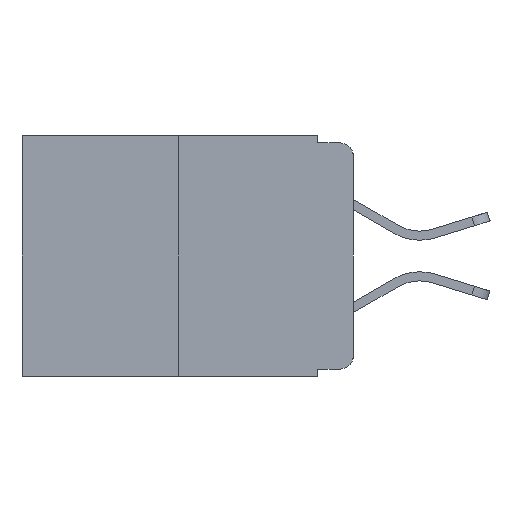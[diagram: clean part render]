
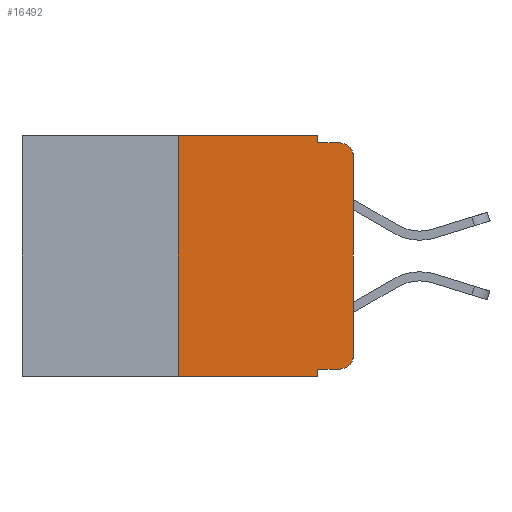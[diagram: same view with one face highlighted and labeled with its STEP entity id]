
A CAD part, left-side view. The second image highlights one B-rep face of the part: STEP entity #16492.
In plain terms, the highlighted planar face has unit normal (-1, 0, 0).
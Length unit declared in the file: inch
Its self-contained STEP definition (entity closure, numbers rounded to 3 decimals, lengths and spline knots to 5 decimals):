
#36 = VERTEX_POINT ( 'NONE', #6370 ) ;
#94 = DIRECTION ( 'NONE',  ( 0., -1., 0. ) ) ;
#273 = LINE ( 'NONE', #22919, #15031 ) ;
#414 = DIRECTION ( 'NONE',  ( 0., 0., 1. ) ) ;
#1648 = EDGE_CURVE ( 'NONE', #11393, #10844, #273, .T. ) ;
#1889 = EDGE_CURVE ( 'NONE', #9114, #8781, #11661, .T. ) ;
#2621 = EDGE_CURVE ( 'NONE', #20983, #8692, #7535, .T. ) ;
#2683 = ORIENTED_EDGE ( 'NONE', *, *, #15283, .F. ) ;
#3445 = PLANE ( 'NONE',  #17469 ) ;
#3870 = CARTESIAN_POINT ( 'NONE',  ( 0., 0.02, -0.333 ) ) ;
#4636 = DIRECTION ( 'NONE',  ( 0., 0., -1. ) ) ;
#5311 = AXIS2_PLACEMENT_3D ( 'NONE', #5682, #7785, #19036 ) ;
#5682 = CARTESIAN_POINT ( 'NONE',  ( 0., 0.02, -0.313 ) ) ;
#5916 = ORIENTED_EDGE ( 'NONE', *, *, #8315, .F. ) ;
#6162 = LINE ( 'NONE', #13438, #12718 ) ;
#6370 = CARTESIAN_POINT ( 'NONE',  ( 0., 0.051, -0.333 ) ) ;
#6625 = EDGE_CURVE ( 'NONE', #36, #10844, #10300, .T. ) ;
#6640 = ORIENTED_EDGE ( 'NONE', *, *, #12602, .F. ) ;
#7273 = CARTESIAN_POINT ( 'NONE',  ( 0., 0.473, 0. ) ) ;
#7356 = CARTESIAN_POINT ( 'NONE',  ( 0., 0.051, -0.01 ) ) ;
#7535 = LINE ( 'NONE', #22982, #11727 ) ;
#7785 = DIRECTION ( 'NONE',  ( -1., 0., 0. ) ) ;
#7858 = CARTESIAN_POINT ( 'NONE',  ( 0., 0., 0. ) ) ;
#7946 = DIRECTION ( 'NONE',  ( 0., -1., 0. ) ) ;
#8080 = ORIENTED_EDGE ( 'NONE', *, *, #1648, .T. ) ;
#8315 = EDGE_CURVE ( 'NONE', #11393, #20983, #23577, .T. ) ;
#8424 = ORIENTED_EDGE ( 'NONE', *, *, #2621, .F. ) ;
#8571 = CARTESIAN_POINT ( 'NONE',  ( 0., 0.051, -0.01 ) ) ;
#8614 = VERTEX_POINT ( 'NONE', #7356 ) ;
#8692 = VERTEX_POINT ( 'NONE', #10287 ) ;
#8781 = VERTEX_POINT ( 'NONE', #16011 ) ;
#9114 = VERTEX_POINT ( 'NONE', #21158 ) ;
#10287 = CARTESIAN_POINT ( 'NONE',  ( 0., 0.051, 0. ) ) ;
#10300 = LINE ( 'NONE', #21579, #15223 ) ;
#10808 = EDGE_CURVE ( 'NONE', #15470, #18124, #13994, .T. ) ;
#10844 = VERTEX_POINT ( 'NONE', #22866 ) ;
#11393 = VERTEX_POINT ( 'NONE', #18338 ) ;
#11661 = CIRCLE ( 'NONE', #14442, 0.02 ) ;
#11727 = VECTOR ( 'NONE', #94, 39.37008 ) ;
#11922 = DIRECTION ( 'NONE',  ( 0., 0., 1. ) ) ;
#12444 = ORIENTED_EDGE ( 'NONE', *, *, #10808, .T. ) ;
#12506 = LINE ( 'NONE', #8571, #15147 ) ;
#12602 = EDGE_CURVE ( 'NONE', #8614, #8781, #12506, .T. ) ;
#12718 = VECTOR ( 'NONE', #17678, 39.37008 ) ;
#12773 = VECTOR ( 'NONE', #414, 39.37008 ) ;
#12774 = DIRECTION ( 'NONE',  ( 0., -1., 0. ) ) ;
#13438 = CARTESIAN_POINT ( 'NONE',  ( 0., 0.051, 0. ) ) ;
#13825 = ORIENTED_EDGE ( 'NONE', *, *, #6625, .F. ) ;
#13994 = CIRCLE ( 'NONE', #5311, 0.02 ) ;
#14346 = CARTESIAN_POINT ( 'NONE',  ( 0., 0.25, 0. ) ) ;
#14442 = AXIS2_PLACEMENT_3D ( 'NONE', #18471, #16737, #18846 ) ;
#14636 = LINE ( 'NONE', #22188, #19195 ) ;
#14823 = DIRECTION ( 'NONE',  ( 1., 0., 0. ) ) ;
#15031 = VECTOR ( 'NONE', #7946, 39.37008 ) ;
#15128 = ORIENTED_EDGE ( 'NONE', *, *, #20516, .T. ) ;
#15147 = VECTOR ( 'NONE', #21792, 39.37008 ) ;
#15223 = VECTOR ( 'NONE', #4636, 39.37008 ) ;
#15283 = EDGE_CURVE ( 'NONE', #8692, #8614, #6162, .T. ) ;
#15311 = DIRECTION ( 'NONE',  ( 0., 0., -1. ) ) ;
#15470 = VERTEX_POINT ( 'NONE', #3870 ) ;
#15535 = LINE ( 'NONE', #7858, #12773 ) ;
#16011 = CARTESIAN_POINT ( 'NONE',  ( 0., 0.02, -0.01 ) ) ;
#16492 = ADVANCED_FACE ( 'NONE', ( #24212 ), #3445, .F. ) ;
#16737 = DIRECTION ( 'NONE',  ( -1., 0., 0. ) ) ;
#17469 = AXIS2_PLACEMENT_3D ( 'NONE', #7273, #14823, #15311 ) ;
#17678 = DIRECTION ( 'NONE',  ( 0., 0., -1. ) ) ;
#18124 = VERTEX_POINT ( 'NONE', #23831 ) ;
#18338 = CARTESIAN_POINT ( 'NONE',  ( 0., 0.25, -0.343 ) ) ;
#18386 = EDGE_CURVE ( 'NONE', #18124, #9114, #15535, .T. ) ;
#18471 = CARTESIAN_POINT ( 'NONE',  ( 0., 0.02, -0.03 ) ) ;
#18846 = DIRECTION ( 'NONE',  ( 0., 0., -1. ) ) ;
#19036 = DIRECTION ( 'NONE',  ( 0., 0., -1. ) ) ;
#19195 = VECTOR ( 'NONE', #12774, 39.37008 ) ;
#19666 = EDGE_LOOP ( 'NONE', ( #22385, #20369, #6640, #2683, #8424, #5916, #8080, #13825, #15128, #12444 ) ) ;
#20369 = ORIENTED_EDGE ( 'NONE', *, *, #1889, .T. ) ;
#20516 = EDGE_CURVE ( 'NONE', #36, #15470, #14636, .T. ) ;
#20983 = VERTEX_POINT ( 'NONE', #14346 ) ;
#21158 = CARTESIAN_POINT ( 'NONE',  ( 0., 0., -0.03 ) ) ;
#21579 = CARTESIAN_POINT ( 'NONE',  ( 0., 0.051, 0. ) ) ;
#21792 = DIRECTION ( 'NONE',  ( 0., -1., 0. ) ) ;
#22188 = CARTESIAN_POINT ( 'NONE',  ( 0., 0.051, -0.333 ) ) ;
#22385 = ORIENTED_EDGE ( 'NONE', *, *, #18386, .T. ) ;
#22460 = VECTOR ( 'NONE', #11922, 39.37008 ) ;
#22866 = CARTESIAN_POINT ( 'NONE',  ( 0., 0.051, -0.343 ) ) ;
#22919 = CARTESIAN_POINT ( 'NONE',  ( 0., 0.473, -0.343 ) ) ;
#22982 = CARTESIAN_POINT ( 'NONE',  ( 0., 0.473, 0. ) ) ;
#23438 = CARTESIAN_POINT ( 'NONE',  ( 0., 0.25, 0. ) ) ;
#23577 = LINE ( 'NONE', #23438, #22460 ) ;
#23831 = CARTESIAN_POINT ( 'NONE',  ( 0., 0., -0.313 ) ) ;
#24212 = FACE_OUTER_BOUND ( 'NONE', #19666, .T. ) ;
